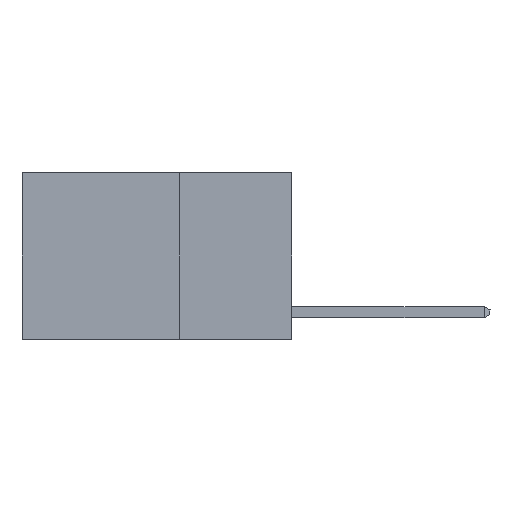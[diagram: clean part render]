
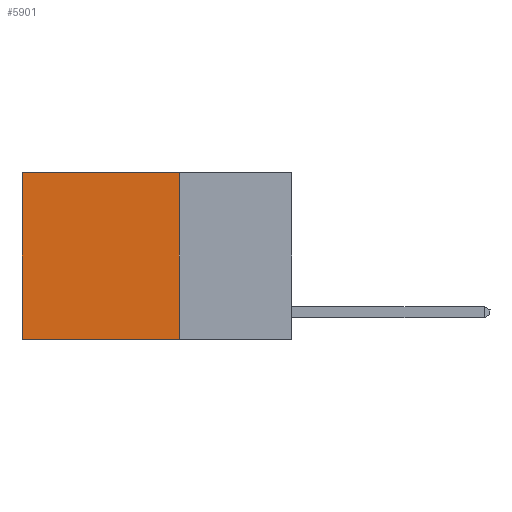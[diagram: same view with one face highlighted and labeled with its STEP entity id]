
A CAD part, left-side view. The second image highlights one B-rep face of the part: STEP entity #5901.
In plain terms, the highlighted planar face has unit normal (-1, 0, 0).
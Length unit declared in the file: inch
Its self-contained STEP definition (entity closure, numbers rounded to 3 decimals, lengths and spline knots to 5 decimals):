
#18 = VERTEX_POINT ( 'NONE', #13384 ) ;
#447 = DIRECTION ( 'NONE',  ( 0., 0., -1. ) ) ;
#517 = ORIENTED_EDGE ( 'NONE', *, *, #7100, .T. ) ;
#1186 = CARTESIAN_POINT ( 'NONE',  ( 0.2625, 0.25, 0. ) ) ;
#1393 = VECTOR ( 'NONE', #4887, 39.37008 ) ;
#1727 = EDGE_CURVE ( 'NONE', #10701, #18, #9589, .T. ) ;
#2842 = CARTESIAN_POINT ( 'NONE',  ( 0.2625, 0.6, 0. ) ) ;
#3350 = DIRECTION ( 'NONE',  ( 0., 1., 0. ) ) ;
#3412 = VECTOR ( 'NONE', #3350, 39.37008 ) ;
#4394 = CARTESIAN_POINT ( 'NONE',  ( 0.2625, 0.25, 0. ) ) ;
#4720 = CARTESIAN_POINT ( 'NONE',  ( 0.2625, 0.25, 0. ) ) ;
#4749 = VERTEX_POINT ( 'NONE', #14407 ) ;
#4887 = DIRECTION ( 'NONE',  ( 0., 1., 0. ) ) ;
#5364 = EDGE_CURVE ( 'NONE', #15108, #10701, #10094, .T. ) ;
#5862 = VECTOR ( 'NONE', #8310, 39.37008 ) ;
#5901 = ADVANCED_FACE ( 'NONE', ( #12964 ), #6189, .F. ) ;
#6189 = PLANE ( 'NONE',  #10998 ) ;
#6612 = LINE ( 'NONE', #4720, #1393 ) ;
#7100 = EDGE_CURVE ( 'NONE', #4749, #18, #7352, .T. ) ;
#7352 = LINE ( 'NONE', #2842, #12553 ) ;
#8310 = DIRECTION ( 'NONE',  ( 0., 0., -1. ) ) ;
#8392 = EDGE_LOOP ( 'NONE', ( #517, #10663, #14569, #13693 ) ) ;
#8613 = CARTESIAN_POINT ( 'NONE',  ( 0.2625, 0.25, 0. ) ) ;
#9589 = LINE ( 'NONE', #14409, #3412 ) ;
#10094 = LINE ( 'NONE', #4394, #5862 ) ;
#10663 = ORIENTED_EDGE ( 'NONE', *, *, #1727, .F. ) ;
#10701 = VERTEX_POINT ( 'NONE', #10873 ) ;
#10873 = CARTESIAN_POINT ( 'NONE',  ( 0.2625, 0.25, -0.37 ) ) ;
#10998 = AXIS2_PLACEMENT_3D ( 'NONE', #1186, #12089, #14581 ) ;
#12089 = DIRECTION ( 'NONE',  ( 1., 0., 0. ) ) ;
#12553 = VECTOR ( 'NONE', #447, 39.37008 ) ;
#12964 = FACE_OUTER_BOUND ( 'NONE', #8392, .T. ) ;
#13384 = CARTESIAN_POINT ( 'NONE',  ( 0.2625, 0.6, -0.37 ) ) ;
#13693 = ORIENTED_EDGE ( 'NONE', *, *, #14343, .T. ) ;
#14343 = EDGE_CURVE ( 'NONE', #15108, #4749, #6612, .T. ) ;
#14407 = CARTESIAN_POINT ( 'NONE',  ( 0.2625, 0.6, 0. ) ) ;
#14409 = CARTESIAN_POINT ( 'NONE',  ( 0.2625, 0.25, -0.37 ) ) ;
#14569 = ORIENTED_EDGE ( 'NONE', *, *, #5364, .F. ) ;
#14581 = DIRECTION ( 'NONE',  ( 0., 0., -1. ) ) ;
#15108 = VERTEX_POINT ( 'NONE', #8613 ) ;
